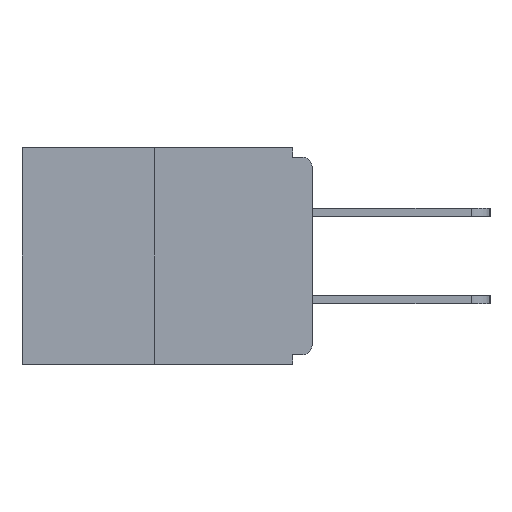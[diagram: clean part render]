
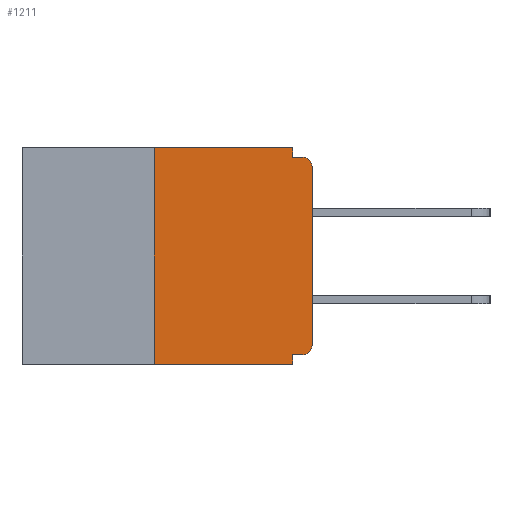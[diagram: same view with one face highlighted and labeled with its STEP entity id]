
A CAD part, left-side view. The second image highlights one B-rep face of the part: STEP entity #1211.
In plain terms, the highlighted planar face has unit normal (-1, 0, 0).
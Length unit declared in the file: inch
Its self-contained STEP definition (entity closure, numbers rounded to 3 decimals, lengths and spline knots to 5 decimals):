
#303 = DIRECTION ( 'NONE',  ( 0., -1., 0. ) ) ;
#597 = CARTESIAN_POINT ( 'NONE',  ( 0., 0.015, -0.03 ) ) ;
#762 = LINE ( 'NONE', #7188, #13077 ) ;
#1211 = ADVANCED_FACE ( 'NONE', ( #16771 ), #11372, .F. ) ;
#1220 = LINE ( 'NONE', #13581, #17135 ) ;
#1243 = CARTESIAN_POINT ( 'NONE',  ( 0., 0.25, 0. ) ) ;
#1459 = EDGE_CURVE ( 'NONE', #16984, #13312, #10948, .T. ) ;
#1965 = DIRECTION ( 'NONE',  ( -1., 0., 0. ) ) ;
#2046 = CIRCLE ( 'NONE', #14374, 0.015 ) ;
#2142 = CARTESIAN_POINT ( 'NONE',  ( 0., 0.015, -0.328 ) ) ;
#2278 = EDGE_CURVE ( 'NONE', #9697, #2364, #6877, .T. ) ;
#2364 = VERTEX_POINT ( 'NONE', #18058 ) ;
#2802 = VERTEX_POINT ( 'NONE', #5836 ) ;
#2840 = VECTOR ( 'NONE', #303, 39.37008 ) ;
#2946 = CARTESIAN_POINT ( 'NONE',  ( 0., 0.25, 0. ) ) ;
#3005 = EDGE_CURVE ( 'NONE', #17128, #9697, #9963, .T. ) ;
#3119 = EDGE_CURVE ( 'NONE', #18515, #16782, #1220, .T. ) ;
#3372 = EDGE_CURVE ( 'NONE', #14821, #2364, #762, .T. ) ;
#4799 = VECTOR ( 'NONE', #7873, 39.37008 ) ;
#5091 = CIRCLE ( 'NONE', #9531, 0.015 ) ;
#5121 = CARTESIAN_POINT ( 'NONE',  ( 0., 0.25, -0.343 ) ) ;
#5326 = VECTOR ( 'NONE', #16582, 39.37008 ) ;
#5340 = VERTEX_POINT ( 'NONE', #5994 ) ;
#5475 = DIRECTION ( 'NONE',  ( 1., 0., 0. ) ) ;
#5493 = CARTESIAN_POINT ( 'NONE',  ( 0., 0.031, -0.343 ) ) ;
#5561 = VECTOR ( 'NONE', #12710, 39.37008 ) ;
#5673 = DIRECTION ( 'NONE',  ( 0., -1., 0. ) ) ;
#5836 = CARTESIAN_POINT ( 'NONE',  ( 0., 0., -0.313 ) ) ;
#5994 = CARTESIAN_POINT ( 'NONE',  ( 0., 0., -0.03 ) ) ;
#6576 = CARTESIAN_POINT ( 'NONE',  ( 0., 0.031, 0. ) ) ;
#6737 = CARTESIAN_POINT ( 'NONE',  ( 0., 0.031, -0.328 ) ) ;
#6877 = LINE ( 'NONE', #5493, #9778 ) ;
#6895 = ORIENTED_EDGE ( 'NONE', *, *, #3119, .F. ) ;
#7071 = EDGE_LOOP ( 'NONE', ( #12279, #10524, #17519, #14877, #18064, #17111, #17653, #14319, #6895, #14544 ) ) ;
#7102 = CARTESIAN_POINT ( 'NONE',  ( 0., 0., 0. ) ) ;
#7188 = CARTESIAN_POINT ( 'NONE',  ( 0., 0.46, -0.343 ) ) ;
#7430 = CARTESIAN_POINT ( 'NONE',  ( 0., 0.015, -0.313 ) ) ;
#7554 = EDGE_CURVE ( 'NONE', #2802, #5340, #17859, .T. ) ;
#7749 = DIRECTION ( 'NONE',  ( 0., 0., -1. ) ) ;
#7799 = DIRECTION ( 'NONE',  ( 0., -1., 0. ) ) ;
#7827 = LINE ( 'NONE', #1243, #5561 ) ;
#7873 = DIRECTION ( 'NONE',  ( 0., 1., 0. ) ) ;
#8675 = VECTOR ( 'NONE', #17181, 39.37008 ) ;
#9175 = CARTESIAN_POINT ( 'NONE',  ( 0., 0., -0.328 ) ) ;
#9531 = AXIS2_PLACEMENT_3D ( 'NONE', #7430, #14345, #17380 ) ;
#9697 = VERTEX_POINT ( 'NONE', #6737 ) ;
#9778 = VECTOR ( 'NONE', #14295, 39.37008 ) ;
#9963 = LINE ( 'NONE', #9175, #4799 ) ;
#9988 = CARTESIAN_POINT ( 'NONE',  ( 0., 0.46, 0. ) ) ;
#10416 = CARTESIAN_POINT ( 'NONE',  ( 0., 0.46, 0. ) ) ;
#10524 = ORIENTED_EDGE ( 'NONE', *, *, #15765, .F. ) ;
#10948 = LINE ( 'NONE', #10416, #2840 ) ;
#11372 = PLANE ( 'NONE',  #13008 ) ;
#12279 = ORIENTED_EDGE ( 'NONE', *, *, #1459, .F. ) ;
#12710 = DIRECTION ( 'NONE',  ( 0., 0., 1. ) ) ;
#13008 = AXIS2_PLACEMENT_3D ( 'NONE', #9988, #5475, #14035 ) ;
#13077 = VECTOR ( 'NONE', #5673, 39.37008 ) ;
#13139 = LINE ( 'NONE', #16643, #5326 ) ;
#13312 = VERTEX_POINT ( 'NONE', #6576 ) ;
#13343 = EDGE_CURVE ( 'NONE', #5340, #16782, #2046, .T. ) ;
#13581 = CARTESIAN_POINT ( 'NONE',  ( 0., 0., -0.015 ) ) ;
#13664 = CARTESIAN_POINT ( 'NONE',  ( 0., 0.015, -0.015 ) ) ;
#14035 = DIRECTION ( 'NONE',  ( 0., 0., -1. ) ) ;
#14295 = DIRECTION ( 'NONE',  ( 0., 0., -1. ) ) ;
#14319 = ORIENTED_EDGE ( 'NONE', *, *, #13343, .T. ) ;
#14345 = DIRECTION ( 'NONE',  ( -1., 0., 0. ) ) ;
#14374 = AXIS2_PLACEMENT_3D ( 'NONE', #597, #1965, #7749 ) ;
#14544 = ORIENTED_EDGE ( 'NONE', *, *, #16312, .F. ) ;
#14821 = VERTEX_POINT ( 'NONE', #5121 ) ;
#14877 = ORIENTED_EDGE ( 'NONE', *, *, #2278, .F. ) ;
#15485 = CARTESIAN_POINT ( 'NONE',  ( 0., 0.031, -0.015 ) ) ;
#15765 = EDGE_CURVE ( 'NONE', #14821, #16984, #7827, .T. ) ;
#16312 = EDGE_CURVE ( 'NONE', #13312, #18515, #13139, .T. ) ;
#16491 = EDGE_CURVE ( 'NONE', #17128, #2802, #5091, .T. ) ;
#16582 = DIRECTION ( 'NONE',  ( 0., 0., -1. ) ) ;
#16643 = CARTESIAN_POINT ( 'NONE',  ( 0., 0.031, 0. ) ) ;
#16771 = FACE_OUTER_BOUND ( 'NONE', #7071, .T. ) ;
#16782 = VERTEX_POINT ( 'NONE', #13664 ) ;
#16984 = VERTEX_POINT ( 'NONE', #2946 ) ;
#17111 = ORIENTED_EDGE ( 'NONE', *, *, #16491, .T. ) ;
#17128 = VERTEX_POINT ( 'NONE', #2142 ) ;
#17135 = VECTOR ( 'NONE', #7799, 39.37008 ) ;
#17181 = DIRECTION ( 'NONE',  ( 0., 0., 1. ) ) ;
#17380 = DIRECTION ( 'NONE',  ( 0., 0., -1. ) ) ;
#17519 = ORIENTED_EDGE ( 'NONE', *, *, #3372, .T. ) ;
#17653 = ORIENTED_EDGE ( 'NONE', *, *, #7554, .T. ) ;
#17859 = LINE ( 'NONE', #7102, #8675 ) ;
#18058 = CARTESIAN_POINT ( 'NONE',  ( 0., 0.031, -0.343 ) ) ;
#18064 = ORIENTED_EDGE ( 'NONE', *, *, #3005, .F. ) ;
#18515 = VERTEX_POINT ( 'NONE', #15485 ) ;
